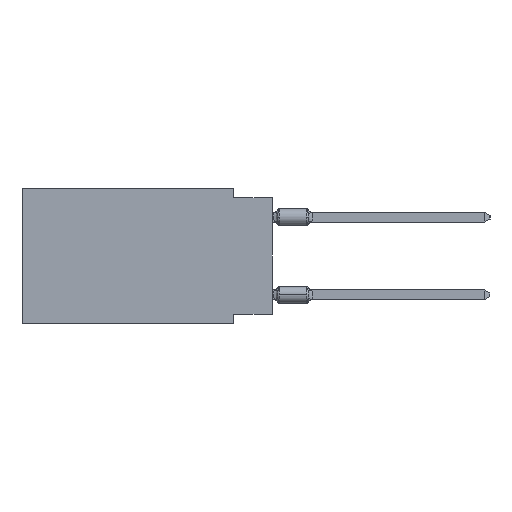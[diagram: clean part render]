
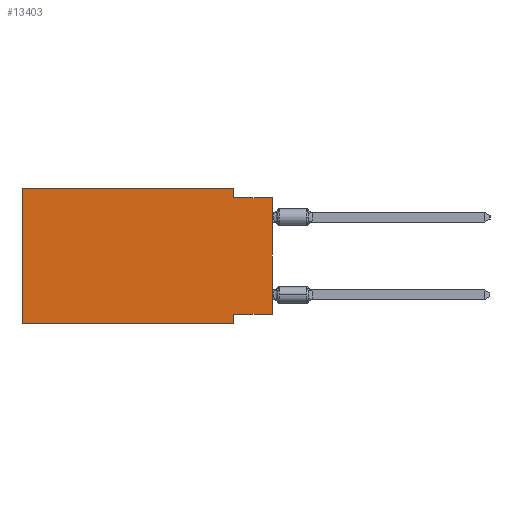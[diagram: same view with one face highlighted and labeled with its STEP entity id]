
A CAD part, left-side view. The second image highlights one B-rep face of the part: STEP entity #13403.
In plain terms, the highlighted planar face has unit normal (-1, 0, 0).
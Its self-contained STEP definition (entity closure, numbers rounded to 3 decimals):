
#957 = LINE ( 'NONE', #32294, #14129 ) ;
#1203 = VERTEX_POINT ( 'NONE', #24463 ) ;
#1293 = DIRECTION ( 'NONE',  ( 0., 1., 0. ) ) ;
#2983 = CARTESIAN_POINT ( 'NONE',  ( 0., 2.54, -8.89 ) ) ;
#2992 = ORIENTED_EDGE ( 'NONE', *, *, #11662, .F. ) ;
#3165 = CARTESIAN_POINT ( 'NONE',  ( 0., 2.54, 0. ) ) ;
#3340 = EDGE_CURVE ( 'NONE', #26471, #1203, #31663, .T. ) ;
#3667 = VERTEX_POINT ( 'NONE', #19293 ) ;
#4416 = ORIENTED_EDGE ( 'NONE', *, *, #9710, .T. ) ;
#4867 = CARTESIAN_POINT ( 'NONE',  ( 0., 0., -0.635 ) ) ;
#5180 = CARTESIAN_POINT ( 'NONE',  ( 0., 16.383, -8.89 ) ) ;
#5822 = AXIS2_PLACEMENT_3D ( 'NONE', #10556, #34169, #19800 ) ;
#6053 = VERTEX_POINT ( 'NONE', #4867 ) ;
#6800 = DIRECTION ( 'NONE',  ( 0., 0., 1. ) ) ;
#7842 = LINE ( 'NONE', #11040, #23840 ) ;
#8404 = DIRECTION ( 'NONE',  ( 0., -1., 0. ) ) ;
#9607 = LINE ( 'NONE', #15625, #31552 ) ;
#9710 = EDGE_CURVE ( 'NONE', #27196, #1203, #10648, .T. ) ;
#10121 = EDGE_CURVE ( 'NONE', #16023, #6053, #24953, .T. ) ;
#10356 = EDGE_CURVE ( 'NONE', #27196, #19661, #957, .T. ) ;
#10406 = DIRECTION ( 'NONE',  ( 0., 0., 1. ) ) ;
#10556 = CARTESIAN_POINT ( 'NONE',  ( 0., 16.383, 0. ) ) ;
#10648 = LINE ( 'NONE', #5180, #12855 ) ;
#10678 = EDGE_CURVE ( 'NONE', #17029, #6053, #13941, .T. ) ;
#11040 = CARTESIAN_POINT ( 'NONE',  ( 0., 16.383, 0. ) ) ;
#11105 = CARTESIAN_POINT ( 'NONE',  ( 0., 0., -0.635 ) ) ;
#11365 = CARTESIAN_POINT ( 'NONE',  ( 0., 0., -8.255 ) ) ;
#11535 = ORIENTED_EDGE ( 'NONE', *, *, #14952, .F. ) ;
#11662 = EDGE_CURVE ( 'NONE', #19661, #3667, #7842, .T. ) ;
#12855 = VECTOR ( 'NONE', #18936, 1000. ) ;
#13403 = ADVANCED_FACE ( 'NONE', ( #16215 ), #28139, .F. ) ;
#13941 = LINE ( 'NONE', #11105, #17734 ) ;
#14129 = VECTOR ( 'NONE', #6800, 1000. ) ;
#14309 = LINE ( 'NONE', #3165, #29193 ) ;
#14421 = CARTESIAN_POINT ( 'NONE',  ( 0., 2.54, -8.255 ) ) ;
#14952 = EDGE_CURVE ( 'NONE', #16023, #26471, #9607, .T. ) ;
#14974 = VECTOR ( 'NONE', #28665, 1000. ) ;
#15625 = CARTESIAN_POINT ( 'NONE',  ( 0., 0., -8.255 ) ) ;
#16023 = VERTEX_POINT ( 'NONE', #11365 ) ;
#16215 = FACE_OUTER_BOUND ( 'NONE', #25205, .T. ) ;
#17029 = VERTEX_POINT ( 'NONE', #21477 ) ;
#17734 = VECTOR ( 'NONE', #23515, 1000. ) ;
#18936 = DIRECTION ( 'NONE',  ( 0., -1., 0. ) ) ;
#19293 = CARTESIAN_POINT ( 'NONE',  ( 0., 2.54, 0. ) ) ;
#19661 = VERTEX_POINT ( 'NONE', #29017 ) ;
#19800 = DIRECTION ( 'NONE',  ( 0., 0., -1. ) ) ;
#20119 = VECTOR ( 'NONE', #10406, 1000. ) ;
#21477 = CARTESIAN_POINT ( 'NONE',  ( 0., 2.54, -0.635 ) ) ;
#22581 = ORIENTED_EDGE ( 'NONE', *, *, #3340, .F. ) ;
#23515 = DIRECTION ( 'NONE',  ( 0., -1., 0. ) ) ;
#23840 = VECTOR ( 'NONE', #8404, 1000. ) ;
#24463 = CARTESIAN_POINT ( 'NONE',  ( 0., 2.54, -8.89 ) ) ;
#24953 = LINE ( 'NONE', #33642, #20119 ) ;
#25025 = CARTESIAN_POINT ( 'NONE',  ( 0., 16.383, -8.89 ) ) ;
#25205 = EDGE_LOOP ( 'NONE', ( #26128, #36082, #27234, #2992, #31364, #4416, #22581, #11535 ) ) ;
#25831 = DIRECTION ( 'NONE',  ( 0., 0., -1. ) ) ;
#26128 = ORIENTED_EDGE ( 'NONE', *, *, #10121, .T. ) ;
#26471 = VERTEX_POINT ( 'NONE', #14421 ) ;
#27196 = VERTEX_POINT ( 'NONE', #25025 ) ;
#27234 = ORIENTED_EDGE ( 'NONE', *, *, #32236, .F. ) ;
#28139 = PLANE ( 'NONE',  #5822 ) ;
#28665 = DIRECTION ( 'NONE',  ( 0., 0., -1. ) ) ;
#29017 = CARTESIAN_POINT ( 'NONE',  ( 0., 16.383, 0. ) ) ;
#29193 = VECTOR ( 'NONE', #25831, 1000. ) ;
#31364 = ORIENTED_EDGE ( 'NONE', *, *, #10356, .F. ) ;
#31552 = VECTOR ( 'NONE', #1293, 1000. ) ;
#31663 = LINE ( 'NONE', #2983, #14974 ) ;
#32236 = EDGE_CURVE ( 'NONE', #3667, #17029, #14309, .T. ) ;
#32294 = CARTESIAN_POINT ( 'NONE',  ( 0., 16.383, 0. ) ) ;
#33642 = CARTESIAN_POINT ( 'NONE',  ( 0., 0., 0. ) ) ;
#34169 = DIRECTION ( 'NONE',  ( 1., 0., 0. ) ) ;
#36082 = ORIENTED_EDGE ( 'NONE', *, *, #10678, .F. ) ;
